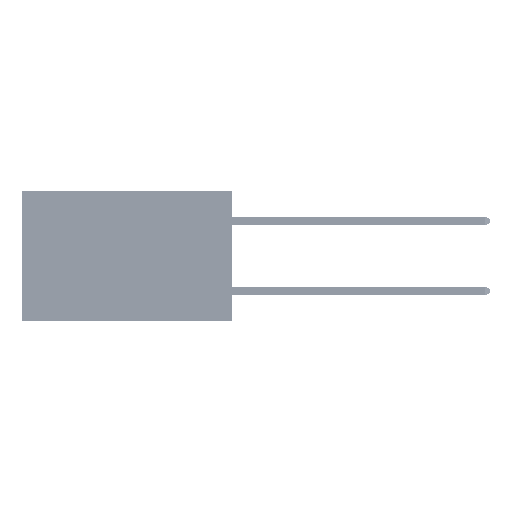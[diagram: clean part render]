
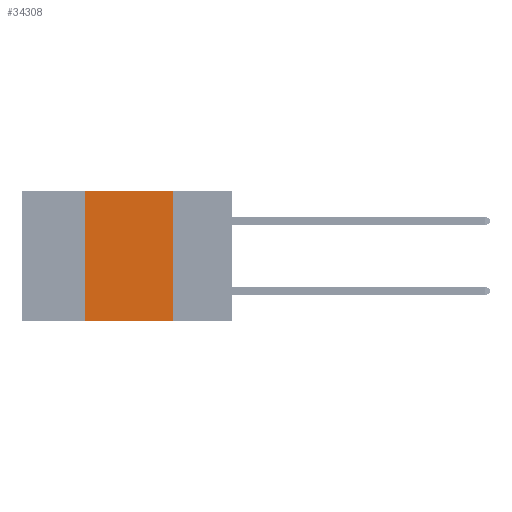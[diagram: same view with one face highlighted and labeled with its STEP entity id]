
A CAD part, left-side view. The second image highlights one B-rep face of the part: STEP entity #34308.
In plain terms, the highlighted planar face has unit normal (-1, 0, 0).
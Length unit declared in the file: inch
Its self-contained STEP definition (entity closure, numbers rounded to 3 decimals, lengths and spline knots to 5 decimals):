
#1574 = VERTEX_POINT ( 'NONE', #10005 ) ;
#1893 = CARTESIAN_POINT ( 'NONE',  ( 0., 0.6, 0. ) ) ;
#3431 = AXIS2_PLACEMENT_3D ( 'NONE', #20957, #35338, #3727 ) ;
#3727 = DIRECTION ( 'NONE',  ( 0., 0., -1. ) ) ;
#4286 = VERTEX_POINT ( 'NONE', #46395 ) ;
#5357 = ORIENTED_EDGE ( 'NONE', *, *, #27287, .F. ) ;
#5424 = LINE ( 'NONE', #1893, #36939 ) ;
#8909 = DIRECTION ( 'NONE',  ( 0., 0., 1. ) ) ;
#10005 = CARTESIAN_POINT ( 'NONE',  ( 0., 0.17, -0.37 ) ) ;
#13311 = LINE ( 'NONE', #45610, #32248 ) ;
#14331 = FACE_OUTER_BOUND ( 'NONE', #39443, .T. ) ;
#15826 = EDGE_CURVE ( 'NONE', #39413, #1574, #13311, .T. ) ;
#19052 = VECTOR ( 'NONE', #40294, 39.37008 ) ;
#19312 = CARTESIAN_POINT ( 'NONE',  ( 0., 0.42, 0. ) ) ;
#20054 = EDGE_CURVE ( 'NONE', #4286, #39413, #5424, .T. ) ;
#20731 = ORIENTED_EDGE ( 'NONE', *, *, #29252, .T. ) ;
#20957 = CARTESIAN_POINT ( 'NONE',  ( 0., 0.6, 0. ) ) ;
#21432 = LINE ( 'NONE', #36525, #19052 ) ;
#23707 = DIRECTION ( 'NONE',  ( 0., 0., -1. ) ) ;
#26151 = LINE ( 'NONE', #19312, #31100 ) ;
#27287 = EDGE_CURVE ( 'NONE', #31605, #4286, #26151, .T. ) ;
#28724 = PLANE ( 'NONE',  #3431 ) ;
#29252 = EDGE_CURVE ( 'NONE', #31605, #1574, #21432, .T. ) ;
#31100 = VECTOR ( 'NONE', #8909, 39.37008 ) ;
#31316 = ORIENTED_EDGE ( 'NONE', *, *, #20054, .F. ) ;
#31605 = VERTEX_POINT ( 'NONE', #33336 ) ;
#32248 = VECTOR ( 'NONE', #23707, 39.37008 ) ;
#33336 = CARTESIAN_POINT ( 'NONE',  ( 0., 0.42, -0.37 ) ) ;
#34295 = CARTESIAN_POINT ( 'NONE',  ( 0., 0.17, 0. ) ) ;
#34308 = ADVANCED_FACE ( 'NONE', ( #14331 ), #28724, .F. ) ;
#35338 = DIRECTION ( 'NONE',  ( 1., 0., 0. ) ) ;
#35550 = ORIENTED_EDGE ( 'NONE', *, *, #15826, .F. ) ;
#36525 = CARTESIAN_POINT ( 'NONE',  ( 0., 0.6, -0.37 ) ) ;
#36939 = VECTOR ( 'NONE', #41037, 39.37008 ) ;
#39413 = VERTEX_POINT ( 'NONE', #34295 ) ;
#39443 = EDGE_LOOP ( 'NONE', ( #35550, #31316, #5357, #20731 ) ) ;
#40294 = DIRECTION ( 'NONE',  ( 0., -1., 0. ) ) ;
#41037 = DIRECTION ( 'NONE',  ( 0., -1., 0. ) ) ;
#45610 = CARTESIAN_POINT ( 'NONE',  ( 0., 0.17, 0. ) ) ;
#46395 = CARTESIAN_POINT ( 'NONE',  ( 0., 0.42, 0. ) ) ;
